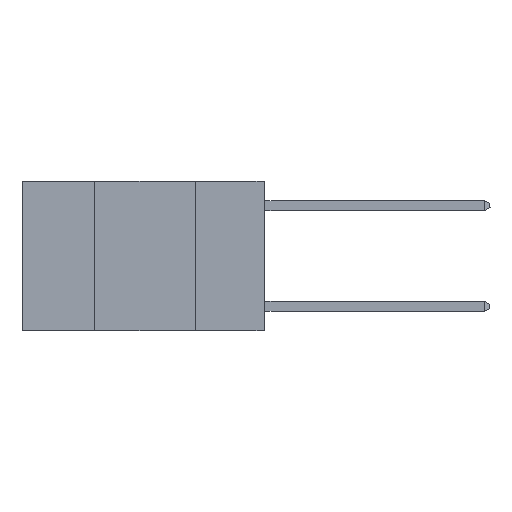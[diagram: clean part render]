
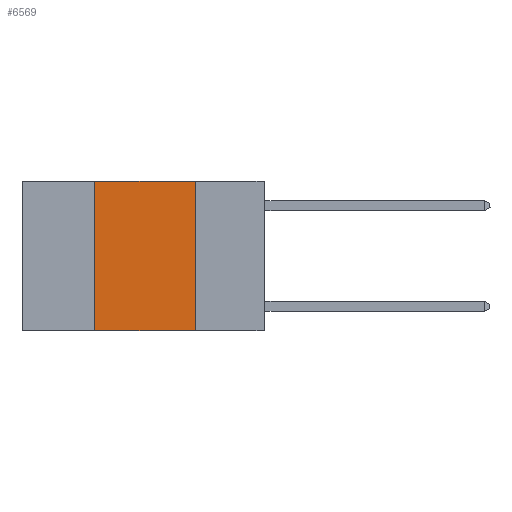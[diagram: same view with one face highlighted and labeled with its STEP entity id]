
A CAD part, left-side view. The second image highlights one B-rep face of the part: STEP entity #6569.
In plain terms, the highlighted planar face has unit normal (-1, 0, 0).
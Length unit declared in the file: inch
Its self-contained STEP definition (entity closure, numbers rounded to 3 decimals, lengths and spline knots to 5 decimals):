
#27 = VERTEX_POINT ( 'NONE', #9774 ) ;
#55 = LINE ( 'NONE', #6420, #8270 ) ;
#91 = DIRECTION ( 'NONE',  ( 0., 0., 1. ) ) ;
#257 = VECTOR ( 'NONE', #2766, 39.37008 ) ;
#533 = LINE ( 'NONE', #4438, #257 ) ;
#541 = DIRECTION ( 'NONE',  ( 0., 0., -1. ) ) ;
#760 = ORIENTED_EDGE ( 'NONE', *, *, #6815, .T. ) ;
#1312 = VECTOR ( 'NONE', #10083, 39.37008 ) ;
#1589 = LINE ( 'NONE', #6258, #1312 ) ;
#2060 = VERTEX_POINT ( 'NONE', #4941 ) ;
#2428 = VERTEX_POINT ( 'NONE', #8456 ) ;
#2482 = DIRECTION ( 'NONE',  ( 0., 0., -1. ) ) ;
#2766 = DIRECTION ( 'NONE',  ( 0., -1., 0. ) ) ;
#3026 = ORIENTED_EDGE ( 'NONE', *, *, #4355, .F. ) ;
#3275 = ORIENTED_EDGE ( 'NONE', *, *, #8561, .F. ) ;
#3560 = AXIS2_PLACEMENT_3D ( 'NONE', #10390, #7366, #2482 ) ;
#4355 = EDGE_CURVE ( 'NONE', #27, #2428, #7110, .T. ) ;
#4438 = CARTESIAN_POINT ( 'NONE',  ( 0., 0.6, -0.37 ) ) ;
#4594 = EDGE_CURVE ( 'NONE', #4698, #2060, #55, .T. ) ;
#4698 = VERTEX_POINT ( 'NONE', #5788 ) ;
#4941 = CARTESIAN_POINT ( 'NONE',  ( 0., 0.17, -0.37 ) ) ;
#5084 = EDGE_LOOP ( 'NONE', ( #7354, #3275, #3026, #760 ) ) ;
#5788 = CARTESIAN_POINT ( 'NONE',  ( 0., 0.17, 0. ) ) ;
#6006 = CARTESIAN_POINT ( 'NONE',  ( 0., 0.42, 0. ) ) ;
#6258 = CARTESIAN_POINT ( 'NONE',  ( 0., 0.6, 0. ) ) ;
#6420 = CARTESIAN_POINT ( 'NONE',  ( 0., 0.17, 0. ) ) ;
#6569 = ADVANCED_FACE ( 'NONE', ( #7055 ), #6578, .F. ) ;
#6578 = PLANE ( 'NONE',  #3560 ) ;
#6815 = EDGE_CURVE ( 'NONE', #27, #2060, #533, .T. ) ;
#6873 = VECTOR ( 'NONE', #91, 39.37008 ) ;
#7055 = FACE_OUTER_BOUND ( 'NONE', #5084, .T. ) ;
#7110 = LINE ( 'NONE', #6006, #6873 ) ;
#7354 = ORIENTED_EDGE ( 'NONE', *, *, #4594, .F. ) ;
#7366 = DIRECTION ( 'NONE',  ( 1., 0., 0. ) ) ;
#8270 = VECTOR ( 'NONE', #541, 39.37008 ) ;
#8456 = CARTESIAN_POINT ( 'NONE',  ( 0., 0.42, 0. ) ) ;
#8561 = EDGE_CURVE ( 'NONE', #2428, #4698, #1589, .T. ) ;
#9774 = CARTESIAN_POINT ( 'NONE',  ( 0., 0.42, -0.37 ) ) ;
#10083 = DIRECTION ( 'NONE',  ( 0., -1., 0. ) ) ;
#10390 = CARTESIAN_POINT ( 'NONE',  ( 0., 0.6, 0. ) ) ;
